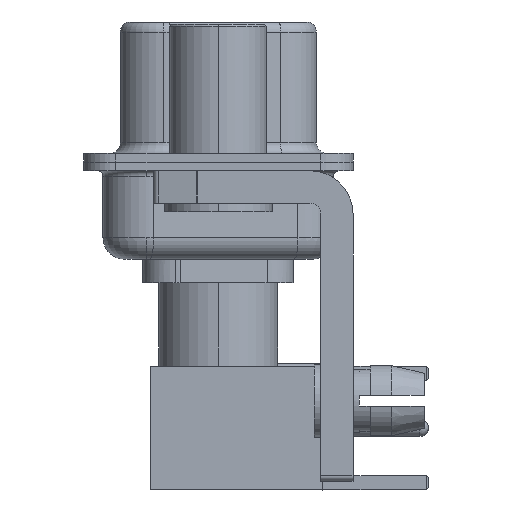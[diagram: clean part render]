
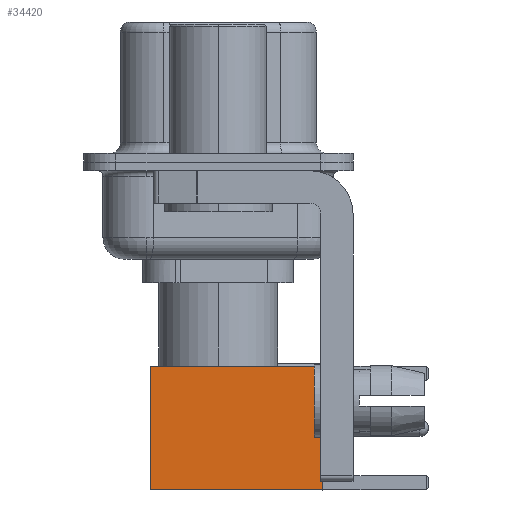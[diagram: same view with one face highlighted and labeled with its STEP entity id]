
A CAD part, left-side view. The second image highlights one B-rep face of the part: STEP entity #34420.
In plain terms, the highlighted face is planar.
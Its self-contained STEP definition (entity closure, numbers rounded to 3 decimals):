
#803 = VECTOR ( 'NONE', #17730, 1000. ) ;
#2253 = DIRECTION ( 'NONE',  ( -1., 0., 0. ) ) ;
#3214 = PLANE ( 'NONE',  #13905 ) ;
#3317 = EDGE_LOOP ( 'NONE', ( #20693, #10803, #8966, #13621 ) ) ;
#3695 = VECTOR ( 'NONE', #2253, 1000. ) ;
#4552 = EDGE_CURVE ( 'NONE', #6096, #28009, #6754, .T. ) ;
#5163 = EDGE_CURVE ( 'NONE', #6096, #20359, #34489, .T. ) ;
#6096 = VERTEX_POINT ( 'NONE', #18776 ) ;
#6754 = LINE ( 'NONE', #28533, #803 ) ;
#8966 = ORIENTED_EDGE ( 'NONE', *, *, #32855, .F. ) ;
#9233 = DIRECTION ( 'NONE',  ( 0., 1., 0. ) ) ;
#10581 = CARTESIAN_POINT ( 'NONE',  ( 0., 2.875, 8. ) ) ;
#10803 = ORIENTED_EDGE ( 'NONE', *, *, #31312, .T. ) ;
#13409 = CARTESIAN_POINT ( 'NONE',  ( 0., 2.875, 0. ) ) ;
#13621 = ORIENTED_EDGE ( 'NONE', *, *, #5163, .F. ) ;
#13757 = DIRECTION ( 'NONE',  ( -1., 0., 0. ) ) ;
#13905 = AXIS2_PLACEMENT_3D ( 'NONE', #14011, #9233, #30302 ) ;
#14011 = CARTESIAN_POINT ( 'NONE',  ( 2.875, 2.875, 0. ) ) ;
#14930 = CARTESIAN_POINT ( 'NONE',  ( -2.875, 2.875, 8. ) ) ;
#15291 = VERTEX_POINT ( 'NONE', #18367 ) ;
#17730 = DIRECTION ( 'NONE',  ( 0., 0., -1. ) ) ;
#18367 = CARTESIAN_POINT ( 'NONE',  ( -2.875, 2.875, 0. ) ) ;
#18776 = CARTESIAN_POINT ( 'NONE',  ( 2.875, 2.875, 8. ) ) ;
#19089 = LINE ( 'NONE', #13409, #20557 ) ;
#19515 = CARTESIAN_POINT ( 'NONE',  ( -2.875, 2.875, 0. ) ) ;
#20359 = VERTEX_POINT ( 'NONE', #14930 ) ;
#20557 = VECTOR ( 'NONE', #13757, 1000. ) ;
#20693 = ORIENTED_EDGE ( 'NONE', *, *, #4552, .T. ) ;
#21183 = VECTOR ( 'NONE', #30475, 1000. ) ;
#22129 = CARTESIAN_POINT ( 'NONE',  ( 2.875, 2.875, 0. ) ) ;
#25183 = FACE_OUTER_BOUND ( 'NONE', #3317, .T. ) ;
#28009 = VERTEX_POINT ( 'NONE', #22129 ) ;
#28533 = CARTESIAN_POINT ( 'NONE',  ( 2.875, 2.875, 0. ) ) ;
#30302 = DIRECTION ( 'NONE',  ( 0., 0., 1. ) ) ;
#30475 = DIRECTION ( 'NONE',  ( 0., 0., -1. ) ) ;
#31312 = EDGE_CURVE ( 'NONE', #28009, #15291, #19089, .T. ) ;
#32855 = EDGE_CURVE ( 'NONE', #20359, #15291, #33310, .T. ) ;
#33310 = LINE ( 'NONE', #19515, #21183 ) ;
#34420 = ADVANCED_FACE ( 'NONE', ( #25183 ), #3214, .T. ) ;
#34489 = LINE ( 'NONE', #10581, #3695 ) ;
